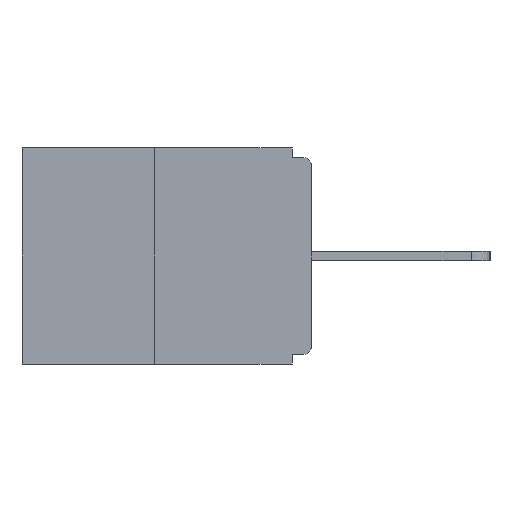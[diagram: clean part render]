
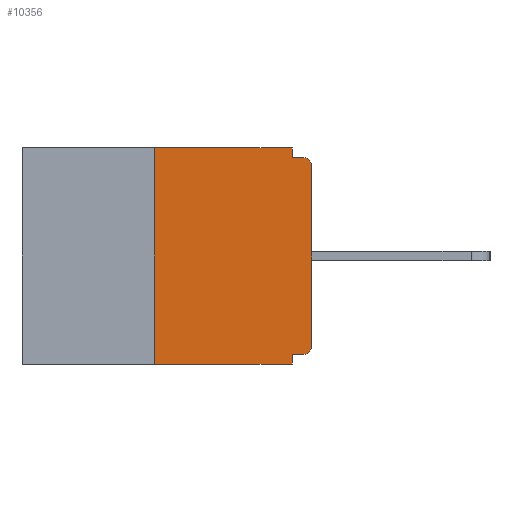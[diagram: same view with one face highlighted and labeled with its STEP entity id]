
A CAD part, left-side view. The second image highlights one B-rep face of the part: STEP entity #10356.
In plain terms, the highlighted planar face has unit normal (-1, 0, 0).
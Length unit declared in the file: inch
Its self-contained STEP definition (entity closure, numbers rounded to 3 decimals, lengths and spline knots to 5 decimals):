
#166 = EDGE_CURVE ( 'NONE', #3468, #7184, #13629, .T. ) ;
#436 = ORIENTED_EDGE ( 'NONE', *, *, #4203, .T. ) ;
#459 = DIRECTION ( 'NONE',  ( 0., 0., -1. ) ) ;
#539 = DIRECTION ( 'NONE',  ( 0., -1., 0. ) ) ;
#638 = EDGE_CURVE ( 'NONE', #9112, #7184, #7005, .T. ) ;
#700 = CARTESIAN_POINT ( 'NONE',  ( 0., 0., -0.328 ) ) ;
#805 = DIRECTION ( 'NONE',  ( -1., 0., 0. ) ) ;
#892 = CARTESIAN_POINT ( 'NONE',  ( 0., 0., -0.313 ) ) ;
#1031 = CARTESIAN_POINT ( 'NONE',  ( 0., 0.015, -0.015 ) ) ;
#1155 = VECTOR ( 'NONE', #539, 39.37008 ) ;
#1210 = DIRECTION ( 'NONE',  ( 0., 0., -1. ) ) ;
#1318 = VERTEX_POINT ( 'NONE', #13613 ) ;
#1428 = VECTOR ( 'NONE', #8859, 39.37008 ) ;
#1666 = CARTESIAN_POINT ( 'NONE',  ( 0., 0.031, 0. ) ) ;
#1897 = DIRECTION ( 'NONE',  ( 0., 0., -1. ) ) ;
#1953 = CARTESIAN_POINT ( 'NONE',  ( 0., 0.46, -0.343 ) ) ;
#2160 = EDGE_CURVE ( 'NONE', #6900, #12607, #10513, .T. ) ;
#2250 = VECTOR ( 'NONE', #9350, 39.37008 ) ;
#2265 = CARTESIAN_POINT ( 'NONE',  ( 0., 0., -0.03 ) ) ;
#2303 = CARTESIAN_POINT ( 'NONE',  ( 0., 0., 0. ) ) ;
#2326 = AXIS2_PLACEMENT_3D ( 'NONE', #3518, #5780, #459 ) ;
#2379 = LINE ( 'NONE', #7717, #2714 ) ;
#2432 = ORIENTED_EDGE ( 'NONE', *, *, #638, .F. ) ;
#2543 = VERTEX_POINT ( 'NONE', #4757 ) ;
#2657 = ORIENTED_EDGE ( 'NONE', *, *, #166, .T. ) ;
#2714 = VECTOR ( 'NONE', #4454, 39.37008 ) ;
#2878 = CARTESIAN_POINT ( 'NONE',  ( 0., 0.25, 0. ) ) ;
#2910 = LINE ( 'NONE', #1666, #2250 ) ;
#2952 = ORIENTED_EDGE ( 'NONE', *, *, #8952, .F. ) ;
#2989 = CIRCLE ( 'NONE', #8901, 0.015 ) ;
#3166 = CARTESIAN_POINT ( 'NONE',  ( 0., 0.031, -0.015 ) ) ;
#3315 = DIRECTION ( 'NONE',  ( 0., -1., 0. ) ) ;
#3468 = VERTEX_POINT ( 'NONE', #2265 ) ;
#3518 = CARTESIAN_POINT ( 'NONE',  ( 0., 0.015, -0.03 ) ) ;
#3553 = DIRECTION ( 'NONE',  ( 0., -1., 0. ) ) ;
#3712 = VECTOR ( 'NONE', #3553, 39.37008 ) ;
#3797 = CARTESIAN_POINT ( 'NONE',  ( 0., 0.031, -0.343 ) ) ;
#4036 = ORIENTED_EDGE ( 'NONE', *, *, #5907, .T. ) ;
#4127 = ORIENTED_EDGE ( 'NONE', *, *, #10438, .T. ) ;
#4203 = EDGE_CURVE ( 'NONE', #11900, #12691, #2989, .T. ) ;
#4454 = DIRECTION ( 'NONE',  ( 0., 0., 1. ) ) ;
#4497 = CARTESIAN_POINT ( 'NONE',  ( 0., 0., -0.015 ) ) ;
#4757 = CARTESIAN_POINT ( 'NONE',  ( 0., 0.25, -0.343 ) ) ;
#4963 = VERTEX_POINT ( 'NONE', #3797 ) ;
#5536 = ORIENTED_EDGE ( 'NONE', *, *, #14004, .F. ) ;
#5674 = CARTESIAN_POINT ( 'NONE',  ( 0., 0.46, 0. ) ) ;
#5780 = DIRECTION ( 'NONE',  ( -1., 0., 0. ) ) ;
#5902 = ORIENTED_EDGE ( 'NONE', *, *, #7818, .F. ) ;
#5907 = EDGE_CURVE ( 'NONE', #2543, #4963, #9131, .T. ) ;
#6073 = EDGE_LOOP ( 'NONE', ( #9621, #5536, #4036, #5902, #9142, #436, #4127, #2657, #2432, #2952 ) ) ;
#6713 = DIRECTION ( 'NONE',  ( 1., 0., 0. ) ) ;
#6900 = VERTEX_POINT ( 'NONE', #2878 ) ;
#6953 = DIRECTION ( 'NONE',  ( 0., 0., 1. ) ) ;
#7005 = LINE ( 'NONE', #4497, #7174 ) ;
#7174 = VECTOR ( 'NONE', #3315, 39.37008 ) ;
#7184 = VERTEX_POINT ( 'NONE', #1031 ) ;
#7199 = LINE ( 'NONE', #7802, #1428 ) ;
#7311 = CARTESIAN_POINT ( 'NONE',  ( 0., 0.015, -0.313 ) ) ;
#7407 = CARTESIAN_POINT ( 'NONE',  ( 0., 0.031, 0. ) ) ;
#7717 = CARTESIAN_POINT ( 'NONE',  ( 0., 0.25, 0. ) ) ;
#7796 = VECTOR ( 'NONE', #6953, 39.37008 ) ;
#7802 = CARTESIAN_POINT ( 'NONE',  ( 0., 0.031, -0.343 ) ) ;
#7818 = EDGE_CURVE ( 'NONE', #1318, #4963, #7199, .T. ) ;
#7887 = AXIS2_PLACEMENT_3D ( 'NONE', #8514, #6713, #1210 ) ;
#8514 = CARTESIAN_POINT ( 'NONE',  ( 0., 0.46, 0. ) ) ;
#8859 = DIRECTION ( 'NONE',  ( 0., 0., -1. ) ) ;
#8901 = AXIS2_PLACEMENT_3D ( 'NONE', #7311, #805, #1897 ) ;
#8952 = EDGE_CURVE ( 'NONE', #12607, #9112, #2910, .T. ) ;
#9112 = VERTEX_POINT ( 'NONE', #3166 ) ;
#9131 = LINE ( 'NONE', #1953, #1155 ) ;
#9142 = ORIENTED_EDGE ( 'NONE', *, *, #10303, .F. ) ;
#9294 = CARTESIAN_POINT ( 'NONE',  ( 0., 0.015, -0.328 ) ) ;
#9350 = DIRECTION ( 'NONE',  ( 0., 0., -1. ) ) ;
#9417 = DIRECTION ( 'NONE',  ( 0., 1., 0. ) ) ;
#9621 = ORIENTED_EDGE ( 'NONE', *, *, #2160, .F. ) ;
#10303 = EDGE_CURVE ( 'NONE', #11900, #1318, #13915, .T. ) ;
#10356 = ADVANCED_FACE ( 'NONE', ( #12579 ), #13994, .F. ) ;
#10438 = EDGE_CURVE ( 'NONE', #12691, #3468, #12383, .T. ) ;
#10513 = LINE ( 'NONE', #5674, #3712 ) ;
#11900 = VERTEX_POINT ( 'NONE', #9294 ) ;
#12383 = LINE ( 'NONE', #2303, #7796 ) ;
#12579 = FACE_OUTER_BOUND ( 'NONE', #6073, .T. ) ;
#12607 = VERTEX_POINT ( 'NONE', #7407 ) ;
#12691 = VERTEX_POINT ( 'NONE', #892 ) ;
#13256 = VECTOR ( 'NONE', #9417, 39.37008 ) ;
#13613 = CARTESIAN_POINT ( 'NONE',  ( 0., 0.031, -0.328 ) ) ;
#13629 = CIRCLE ( 'NONE', #2326, 0.015 ) ;
#13915 = LINE ( 'NONE', #700, #13256 ) ;
#13994 = PLANE ( 'NONE',  #7887 ) ;
#14004 = EDGE_CURVE ( 'NONE', #2543, #6900, #2379, .T. ) ;
